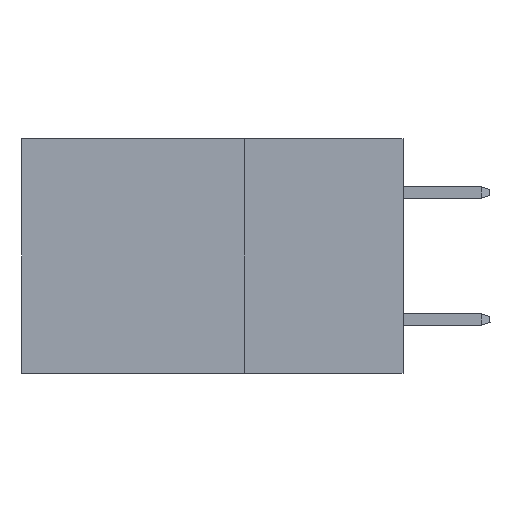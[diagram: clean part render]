
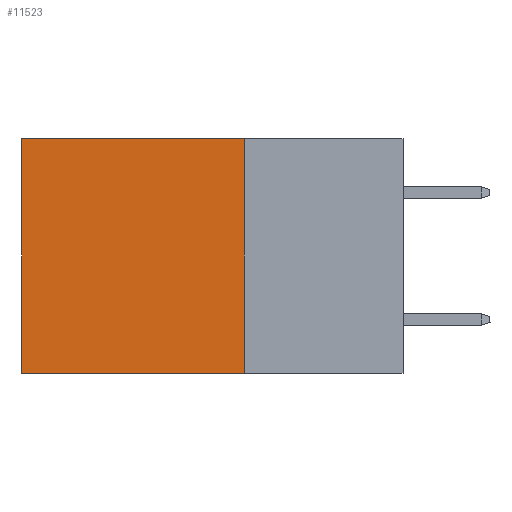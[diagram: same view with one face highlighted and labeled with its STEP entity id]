
A CAD part, left-side view. The second image highlights one B-rep face of the part: STEP entity #11523.
In plain terms, the highlighted planar face has unit normal (-1, 0, 0).
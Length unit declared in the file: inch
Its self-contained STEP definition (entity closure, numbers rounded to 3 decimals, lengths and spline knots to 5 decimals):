
#879 = CARTESIAN_POINT ( 'NONE',  ( 0.2875, 0.25, -0.37 ) ) ;
#2057 = FACE_OUTER_BOUND ( 'NONE', #4144, .T. ) ;
#2102 = EDGE_CURVE ( 'NONE', #12174, #2530, #6747, .T. ) ;
#2530 = VERTEX_POINT ( 'NONE', #879 ) ;
#4144 = EDGE_LOOP ( 'NONE', ( #5513, #21268, #6078, #7302 ) ) ;
#5425 = EDGE_CURVE ( 'NONE', #22880, #5470, #11781, .T. ) ;
#5470 = VERTEX_POINT ( 'NONE', #23170 ) ;
#5513 = ORIENTED_EDGE ( 'NONE', *, *, #5425, .T. ) ;
#5786 = LINE ( 'NONE', #18788, #6941 ) ;
#6078 = ORIENTED_EDGE ( 'NONE', *, *, #2102, .F. ) ;
#6744 = LINE ( 'NONE', #21767, #8971 ) ;
#6747 = LINE ( 'NONE', #21652, #14976 ) ;
#6941 = VECTOR ( 'NONE', #7861, 39.37008 ) ;
#7302 = ORIENTED_EDGE ( 'NONE', *, *, #7909, .T. ) ;
#7861 = DIRECTION ( 'NONE',  ( 0., 1., 0. ) ) ;
#7909 = EDGE_CURVE ( 'NONE', #12174, #22880, #6744, .T. ) ;
#8457 = DIRECTION ( 'NONE',  ( 0., 0., -1. ) ) ;
#8971 = VECTOR ( 'NONE', #23588, 39.37008 ) ;
#9335 = VECTOR ( 'NONE', #21344, 39.37008 ) ;
#11045 = CARTESIAN_POINT ( 'NONE',  ( 0.2875, 0.25, 0. ) ) ;
#11523 = ADVANCED_FACE ( 'NONE', ( #2057 ), #15045, .F. ) ;
#11781 = LINE ( 'NONE', #11906, #9335 ) ;
#11906 = CARTESIAN_POINT ( 'NONE',  ( 0.2875, 0.6, 0. ) ) ;
#12174 = VERTEX_POINT ( 'NONE', #19739 ) ;
#14932 = DIRECTION ( 'NONE',  ( 1., 0., 0. ) ) ;
#14976 = VECTOR ( 'NONE', #8457, 39.37008 ) ;
#15045 = PLANE ( 'NONE',  #17378 ) ;
#17378 = AXIS2_PLACEMENT_3D ( 'NONE', #11045, #14932, #22193 ) ;
#18482 = EDGE_CURVE ( 'NONE', #2530, #5470, #5786, .T. ) ;
#18788 = CARTESIAN_POINT ( 'NONE',  ( 0.2875, 0.25, -0.37 ) ) ;
#18909 = CARTESIAN_POINT ( 'NONE',  ( 0.2875, 0.6, 0. ) ) ;
#19739 = CARTESIAN_POINT ( 'NONE',  ( 0.2875, 0.25, 0. ) ) ;
#21268 = ORIENTED_EDGE ( 'NONE', *, *, #18482, .F. ) ;
#21344 = DIRECTION ( 'NONE',  ( 0., 0., -1. ) ) ;
#21652 = CARTESIAN_POINT ( 'NONE',  ( 0.2875, 0.25, 0. ) ) ;
#21767 = CARTESIAN_POINT ( 'NONE',  ( 0.2875, 0.25, 0. ) ) ;
#22193 = DIRECTION ( 'NONE',  ( 0., 0., -1. ) ) ;
#22880 = VERTEX_POINT ( 'NONE', #18909 ) ;
#23170 = CARTESIAN_POINT ( 'NONE',  ( 0.2875, 0.6, -0.37 ) ) ;
#23588 = DIRECTION ( 'NONE',  ( 0., 1., 0. ) ) ;
